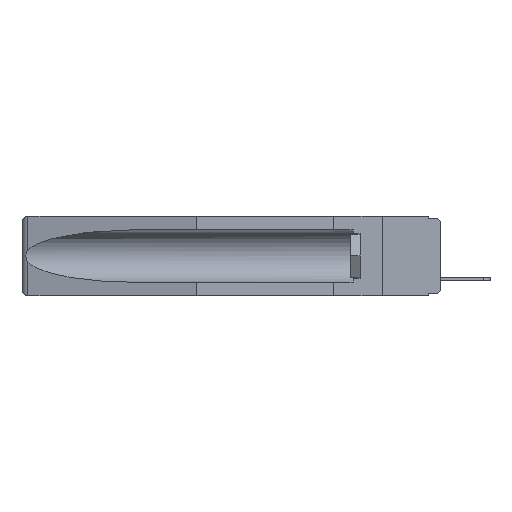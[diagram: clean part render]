
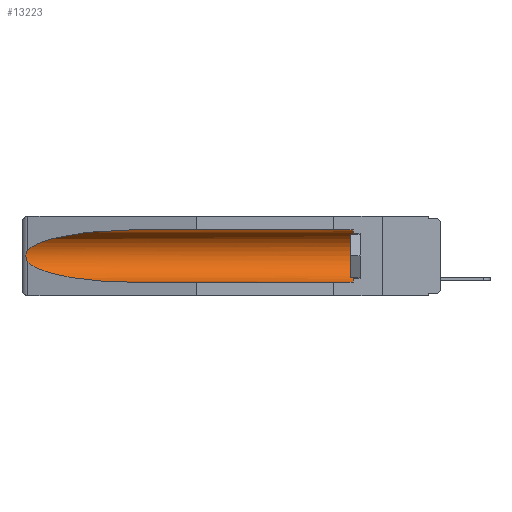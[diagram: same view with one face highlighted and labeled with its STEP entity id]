
A CAD part, left-side view. The second image highlights one B-rep face of the part: STEP entity #13223.
In plain terms, the highlighted cylindrical face has radius 2.857 mm (diameter 5.715 mm), a partial arc.
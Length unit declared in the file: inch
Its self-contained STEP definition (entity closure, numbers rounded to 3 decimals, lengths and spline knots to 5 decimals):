
#32 = CYLINDRICAL_SURFACE ( 'NONE', #2499, 0.1125 ) ;
#103 = CARTESIAN_POINT ( 'NONE',  ( 0.21114, 1.30732, -0.059 ) ) ;
#463 = VERTEX_POINT ( 'NONE', #2205 ) ;
#488 = CARTESIAN_POINT ( 'NONE',  ( 0.2675, 1.53308, -0.17534 ) ) ;
#499 = EDGE_CURVE ( 'NONE', #13819, #6695, #21397, .T. ) ;
#1333 = CARTESIAN_POINT ( 'NONE',  ( 0.26537, 1.52718, -0.14972 ) ) ;
#2205 = CARTESIAN_POINT ( 'NONE',  ( 0.155, 0.126, -0.284 ) ) ;
#2499 = AXIS2_PLACEMENT_3D ( 'NONE', #10465, #16236, #4158 ) ;
#3465 = CARTESIAN_POINT ( 'NONE',  ( 0.155, -0.30754, -0.059 ) ) ;
#3981 =( BOUNDED_CURVE ( )  B_SPLINE_CURVE ( 3, ( #4063, #103, #24310, #18306 ),
 .UNSPECIFIED., .F., .F. ) 
 B_SPLINE_CURVE_WITH_KNOTS ( ( 4, 4 ),
 ( 4.71239, 6.08839 ),
 .UNSPECIFIED. ) 
 CURVE ( )  GEOMETRIC_REPRESENTATION_ITEM ( )  RATIONAL_B_SPLINE_CURVE ( ( 1., 0.848, 0.848, 1. ) ) 
 REPRESENTATION_ITEM ( '' )  );
#4063 = CARTESIAN_POINT ( 'NONE',  ( 0.155, 1.07973, -0.059 ) ) ;
#4141 = CARTESIAN_POINT ( 'NONE',  ( 0.155, 1.07973, -0.284 ) ) ;
#4158 = DIRECTION ( 'NONE',  ( 0., 0., 1. ) ) ;
#4419 = CARTESIAN_POINT ( 'NONE',  ( 0.2673, 1.5327, -0.16383 ) ) ;
#6439 = CARTESIAN_POINT ( 'NONE',  ( 0.2675, 1.53308, -0.16763 ) ) ;
#6462 = VERTEX_POINT ( 'NONE', #14218 ) ;
#6559 = LINE ( 'NONE', #3465, #16391 ) ;
#6614 = CARTESIAN_POINT ( 'NONE',  ( 0.26655, 1.53094, -0.18657 ) ) ;
#6677 = CARTESIAN_POINT ( 'NONE',  ( 0.155, 1.07973, -0.284 ) ) ;
#6695 = VERTEX_POINT ( 'NONE', #6677 ) ;
#6868 = CARTESIAN_POINT ( 'NONE',  ( 0.155, 0.126, -0.059 ) ) ;
#8111 = CARTESIAN_POINT ( 'NONE',  ( 0.21114, 1.30732, -0.284 ) ) ;
#9009 = ORIENTED_EDGE ( 'NONE', *, *, #499, .T. ) ;
#9312 = ORIENTED_EDGE ( 'NONE', *, *, #17304, .T. ) ;
#10028 = EDGE_CURVE ( 'NONE', #15013, #13819, #15272, .T. ) ;
#10465 = CARTESIAN_POINT ( 'NONE',  ( 0.155, -0.30754, -0.1715 ) ) ;
#10586 = CARTESIAN_POINT ( 'NONE',  ( 0.2673, 1.53269, -0.17917 ) ) ;
#11180 = AXIS2_PLACEMENT_3D ( 'NONE', #16923, #22945, #24955 ) ;
#11542 = DIRECTION ( 'NONE',  ( 0., 1., 0. ) ) ;
#12445 = CARTESIAN_POINT ( 'NONE',  ( 0.26537, 1.52718, -0.14972 ) ) ;
#13048 = ORIENTED_EDGE ( 'NONE', *, *, #24233, .F. ) ;
#13223 = ADVANCED_FACE ( 'NONE', ( #20151 ), #32, .F. ) ;
#13627 = EDGE_CURVE ( 'NONE', #23859, #6462, #6559, .T. ) ;
#13819 = VERTEX_POINT ( 'NONE', #18910 ) ;
#14204 = EDGE_LOOP ( 'NONE', ( #9312, #23692, #9009, #13048, #20987, #14493 ) ) ;
#14218 = CARTESIAN_POINT ( 'NONE',  ( 0.155, 1.07973, -0.059 ) ) ;
#14493 = ORIENTED_EDGE ( 'NONE', *, *, #13627, .T. ) ;
#14502 = CARTESIAN_POINT ( 'NONE',  ( 0.26597, 1.52961, -0.15275 ) ) ;
#14582 = CARTESIAN_POINT ( 'NONE',  ( 0.26597, 1.5296, -0.19026 ) ) ;
#14715 = CARTESIAN_POINT ( 'NONE',  ( 0.155, -0.30754, -0.284 ) ) ;
#14736 = CIRCLE ( 'NONE', #11180, 0.1125 ) ;
#15013 = VERTEX_POINT ( 'NONE', #1333 ) ;
#15272 = B_SPLINE_CURVE_WITH_KNOTS ( 'NONE', 3,
 ( #12445, #14502, #16520, #4419, #6439, #488, #10586, #6614, #14582, #22699 ),
 .UNSPECIFIED., .F., .F.,
 ( 4, 2, 2, 2, 4 ),
 ( 0., 0.00029, 0.00058, 0.00087, 0.00117 ),
 .UNSPECIFIED. ) ;
#16236 = DIRECTION ( 'NONE',  ( 0., 1., 0. ) ) ;
#16391 = VECTOR ( 'NONE', #11542, 39.37008 ) ;
#16520 = CARTESIAN_POINT ( 'NONE',  ( 0.26654, 1.53092, -0.15636 ) ) ;
#16677 = EDGE_CURVE ( 'NONE', #463, #23859, #14736, .T. ) ;
#16738 = DIRECTION ( 'NONE',  ( 0., 1., 0. ) ) ;
#16923 = CARTESIAN_POINT ( 'NONE',  ( 0.155, 0.126, -0.1715 ) ) ;
#17304 = EDGE_CURVE ( 'NONE', #6462, #15013, #3981, .T. ) ;
#18306 = CARTESIAN_POINT ( 'NONE',  ( 0.26537, 1.52718, -0.14972 ) ) ;
#18350 = VECTOR ( 'NONE', #16738, 39.37008 ) ;
#18910 = CARTESIAN_POINT ( 'NONE',  ( 0.26537, 1.52718, -0.19328 ) ) ;
#20151 = FACE_OUTER_BOUND ( 'NONE', #14204, .T. ) ;
#20227 = CARTESIAN_POINT ( 'NONE',  ( 0.25451, 1.48313, -0.24835 ) ) ;
#20987 = ORIENTED_EDGE ( 'NONE', *, *, #16677, .T. ) ;
#21397 =( BOUNDED_CURVE ( )  B_SPLINE_CURVE ( 3, ( #23991, #20227, #8111, #4141 ),
 .UNSPECIFIED., .F., .F. ) 
 B_SPLINE_CURVE_WITH_KNOTS ( ( 4, 4 ),
 ( 0.1948, 1.5708 ),
 .UNSPECIFIED. ) 
 CURVE ( )  GEOMETRIC_REPRESENTATION_ITEM ( )  RATIONAL_B_SPLINE_CURVE ( ( 1., 0.848, 0.848, 1. ) ) 
 REPRESENTATION_ITEM ( '' )  );
#22699 = CARTESIAN_POINT ( 'NONE',  ( 0.26537, 1.52718, -0.19328 ) ) ;
#22945 = DIRECTION ( 'NONE',  ( 0., -1., 0. ) ) ;
#23669 = LINE ( 'NONE', #14715, #18350 ) ;
#23692 = ORIENTED_EDGE ( 'NONE', *, *, #10028, .T. ) ;
#23859 = VERTEX_POINT ( 'NONE', #6868 ) ;
#23991 = CARTESIAN_POINT ( 'NONE',  ( 0.26537, 1.52718, -0.19328 ) ) ;
#24233 = EDGE_CURVE ( 'NONE', #463, #6695, #23669, .T. ) ;
#24310 = CARTESIAN_POINT ( 'NONE',  ( 0.25451, 1.48313, -0.09465 ) ) ;
#24955 = DIRECTION ( 'NONE',  ( 0., 0., 1. ) ) ;
